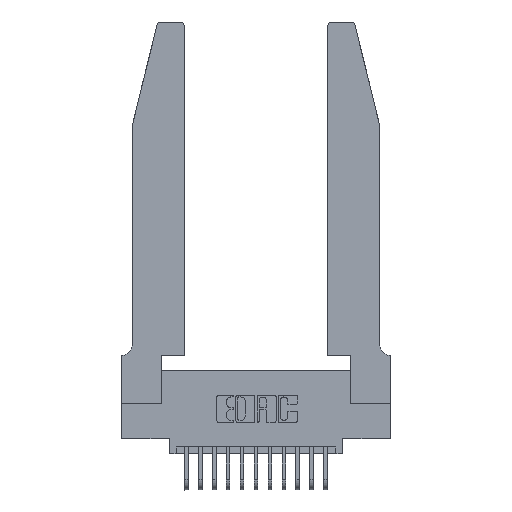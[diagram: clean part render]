
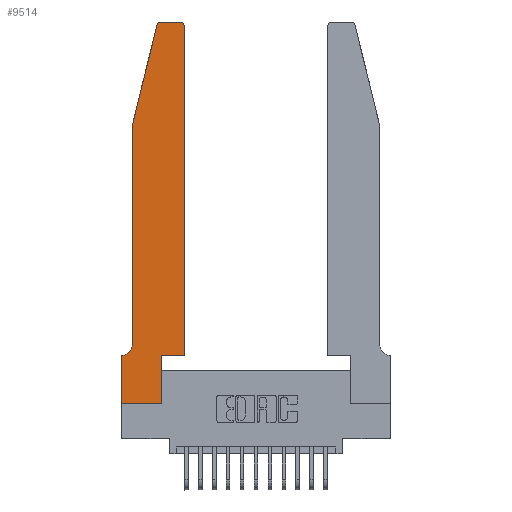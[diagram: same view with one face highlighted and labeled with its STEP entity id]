
A CAD part, top view. The second image highlights one B-rep face of the part: STEP entity #9514.
In plain terms, the highlighted planar face has unit normal (0, 0, 1).
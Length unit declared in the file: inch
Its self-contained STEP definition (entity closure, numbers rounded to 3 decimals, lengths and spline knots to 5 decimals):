
#57 = CARTESIAN_POINT ( 'NONE',  ( 0., 0.35, 0.37 ) ) ;
#162 = DIRECTION ( 'NONE',  ( -1., 0., 0. ) ) ;
#313 = DIRECTION ( 'NONE',  ( -1., 0., 0. ) ) ;
#347 = LINE ( 'NONE', #4249, #14261 ) ;
#365 = LINE ( 'NONE', #11303, #13881 ) ;
#577 = ORIENTED_EDGE ( 'NONE', *, *, #5389, .T. ) ;
#688 = VERTEX_POINT ( 'NONE', #758 ) ;
#758 = CARTESIAN_POINT ( 'NONE',  ( 0.25487, 2.72718, 0.37 ) ) ;
#914 = CARTESIAN_POINT ( 'NONE',  ( 0., 0.35, 0.37 ) ) ;
#1864 = DIRECTION ( 'NONE',  ( 0., 1., 0. ) ) ;
#2191 = DIRECTION ( 'NONE',  ( 1., 0., 0. ) ) ;
#2201 = VERTEX_POINT ( 'NONE', #914 ) ;
#2519 = EDGE_CURVE ( 'NONE', #2723, #14348, #15535, .T. ) ;
#2686 = CARTESIAN_POINT ( 'NONE',  ( 0.2865, 0., 0.37 ) ) ;
#2692 = EDGE_CURVE ( 'NONE', #10596, #12960, #13452, .T. ) ;
#2723 = VERTEX_POINT ( 'NONE', #11677 ) ;
#2841 = ORIENTED_EDGE ( 'NONE', *, *, #2692, .T. ) ;
#3244 = DIRECTION ( 'NONE',  ( 1., 0., 0. ) ) ;
#3779 = CARTESIAN_POINT ( 'NONE',  ( 0.0755, 2., 0.37 ) ) ;
#3827 = LINE ( 'NONE', #8860, #7052 ) ;
#4249 = CARTESIAN_POINT ( 'NONE',  ( 0.2605, 2.75, 0.37 ) ) ;
#4442 = ORIENTED_EDGE ( 'NONE', *, *, #15989, .T. ) ;
#4568 = CARTESIAN_POINT ( 'NONE',  ( 0.284, 2.75, 0.37 ) ) ;
#4764 = ORIENTED_EDGE ( 'NONE', *, *, #11106, .T. ) ;
#4936 = VECTOR ( 'NONE', #9776, 39.37008 ) ;
#5120 = ORIENTED_EDGE ( 'NONE', *, *, #11467, .T. ) ;
#5389 = EDGE_CURVE ( 'NONE', #12249, #6618, #14759, .T. ) ;
#5403 = CARTESIAN_POINT ( 'NONE',  ( 0.0755, 0.35, 0.37 ) ) ;
#5592 = CIRCLE ( 'NONE', #12190, 0.03 ) ;
#5595 = PLANE ( 'NONE',  #9430 ) ;
#5947 = CARTESIAN_POINT ( 'NONE',  ( 0.4505, 0.35, 0.37 ) ) ;
#5965 = CARTESIAN_POINT ( 'NONE',  ( 0.4205, 2.72, 0.37 ) ) ;
#6229 = DIRECTION ( 'NONE',  ( -0.239, -0.971, 0. ) ) ;
#6618 = VERTEX_POINT ( 'NONE', #15175 ) ;
#6937 = VERTEX_POINT ( 'NONE', #14624 ) ;
#6944 = DIRECTION ( 'NONE',  ( 1., 0., 0. ) ) ;
#7052 = VECTOR ( 'NONE', #6229, 39.37008 ) ;
#7327 = ORIENTED_EDGE ( 'NONE', *, *, #11473, .T. ) ;
#7336 = DIRECTION ( 'NONE',  ( 1., 0., 0. ) ) ;
#7689 = CARTESIAN_POINT ( 'NONE',  ( 0.284, 2.72, 0.37 ) ) ;
#7797 = VECTOR ( 'NONE', #13387, 39.37008 ) ;
#8070 = EDGE_CURVE ( 'NONE', #12960, #16062, #365, .T. ) ;
#8407 = AXIS2_PLACEMENT_3D ( 'NONE', #16445, #8474, #313 ) ;
#8474 = DIRECTION ( 'NONE',  ( 0., 0., -1. ) ) ;
#8486 = EDGE_CURVE ( 'NONE', #6937, #13561, #347, .T. ) ;
#8834 = ORIENTED_EDGE ( 'NONE', *, *, #13953, .T. ) ;
#8860 = CARTESIAN_POINT ( 'NONE',  ( 0.0755, 2., 0.37 ) ) ;
#9004 = DIRECTION ( 'NONE',  ( 1., 0., 0. ) ) ;
#9334 = VECTOR ( 'NONE', #13167, 39.37008 ) ;
#9430 = AXIS2_PLACEMENT_3D ( 'NONE', #57, #14901, #6944 ) ;
#9514 = ADVANCED_FACE ( 'NONE', ( #17338 ), #5595, .T. ) ;
#9776 = DIRECTION ( 'NONE',  ( 0., -1., 0. ) ) ;
#10103 = AXIS2_PLACEMENT_3D ( 'NONE', #5965, #15278, #7336 ) ;
#10368 = LINE ( 'NONE', #11309, #17446 ) ;
#10596 = VERTEX_POINT ( 'NONE', #13144 ) ;
#10780 = CIRCLE ( 'NONE', #10103, 0.03 ) ;
#11106 = EDGE_CURVE ( 'NONE', #13561, #688, #5592, .T. ) ;
#11114 = ORIENTED_EDGE ( 'NONE', *, *, #8070, .T. ) ;
#11303 = CARTESIAN_POINT ( 'NONE',  ( 0.2865, 0.35, 0.37 ) ) ;
#11309 = CARTESIAN_POINT ( 'NONE',  ( 0.4505, 0.35, 0.37 ) ) ;
#11333 = CARTESIAN_POINT ( 'NONE',  ( 0.0055, 0.35, 0.37 ) ) ;
#11365 = EDGE_CURVE ( 'NONE', #2201, #10596, #15582, .T. ) ;
#11467 = EDGE_CURVE ( 'NONE', #6618, #6937, #10780, .T. ) ;
#11473 = EDGE_CURVE ( 'NONE', #16062, #12249, #10368, .T. ) ;
#11676 = CARTESIAN_POINT ( 'NONE',  ( 0.2865, 0.35, 0.37 ) ) ;
#11677 = CARTESIAN_POINT ( 'NONE',  ( 0.0755, 0.42, 0.37 ) ) ;
#11725 = EDGE_CURVE ( 'NONE', #14989, #2723, #12855, .T. ) ;
#12190 = AXIS2_PLACEMENT_3D ( 'NONE', #7689, #16966, #9004 ) ;
#12240 = EDGE_LOOP ( 'NONE', ( #14316, #4764, #4442, #16666, #13961, #8834, #16413, #2841, #11114, #7327, #577, #5120 ) ) ;
#12249 = VERTEX_POINT ( 'NONE', #13338 ) ;
#12855 = LINE ( 'NONE', #3779, #9334 ) ;
#12960 = VERTEX_POINT ( 'NONE', #2686 ) ;
#12968 = CARTESIAN_POINT ( 'NONE',  ( 0., 0., 0.37 ) ) ;
#13011 = VECTOR ( 'NONE', #2191, 39.37008 ) ;
#13144 = CARTESIAN_POINT ( 'NONE',  ( 0., 0., 0.37 ) ) ;
#13167 = DIRECTION ( 'NONE',  ( 0., -1., 0. ) ) ;
#13338 = CARTESIAN_POINT ( 'NONE',  ( 0.4505, 0.35, 0.37 ) ) ;
#13387 = DIRECTION ( 'NONE',  ( -1., 0., 0. ) ) ;
#13452 = LINE ( 'NONE', #12968, #13011 ) ;
#13561 = VERTEX_POINT ( 'NONE', #4568 ) ;
#13881 = VECTOR ( 'NONE', #15328, 39.37008 ) ;
#13953 = EDGE_CURVE ( 'NONE', #14348, #2201, #14852, .T. ) ;
#13961 = ORIENTED_EDGE ( 'NONE', *, *, #2519, .T. ) ;
#14261 = VECTOR ( 'NONE', #162, 39.37008 ) ;
#14285 = CARTESIAN_POINT ( 'NONE',  ( 0.0755, 2., 0.37 ) ) ;
#14316 = ORIENTED_EDGE ( 'NONE', *, *, #8486, .T. ) ;
#14335 = VECTOR ( 'NONE', #1864, 39.37008 ) ;
#14348 = VERTEX_POINT ( 'NONE', #11333 ) ;
#14624 = CARTESIAN_POINT ( 'NONE',  ( 0.4205, 2.75, 0.37 ) ) ;
#14759 = LINE ( 'NONE', #5947, #14335 ) ;
#14852 = LINE ( 'NONE', #5403, #7797 ) ;
#14901 = DIRECTION ( 'NONE',  ( 0., 0., 1. ) ) ;
#14989 = VERTEX_POINT ( 'NONE', #14285 ) ;
#15175 = CARTESIAN_POINT ( 'NONE',  ( 0.4505, 2.72, 0.37 ) ) ;
#15278 = DIRECTION ( 'NONE',  ( 0., 0., 1. ) ) ;
#15328 = DIRECTION ( 'NONE',  ( 0., 1., 0. ) ) ;
#15535 = CIRCLE ( 'NONE', #8407, 0.07 ) ;
#15582 = LINE ( 'NONE', #16405, #4936 ) ;
#15989 = EDGE_CURVE ( 'NONE', #688, #14989, #3827, .T. ) ;
#16062 = VERTEX_POINT ( 'NONE', #11676 ) ;
#16405 = CARTESIAN_POINT ( 'NONE',  ( 0., 0., 0.37 ) ) ;
#16413 = ORIENTED_EDGE ( 'NONE', *, *, #11365, .T. ) ;
#16445 = CARTESIAN_POINT ( 'NONE',  ( 0.0055, 0.42, 0.37 ) ) ;
#16666 = ORIENTED_EDGE ( 'NONE', *, *, #11725, .T. ) ;
#16966 = DIRECTION ( 'NONE',  ( 0., 0., 1. ) ) ;
#17338 = FACE_OUTER_BOUND ( 'NONE', #12240, .T. ) ;
#17446 = VECTOR ( 'NONE', #3244, 39.37008 ) ;
